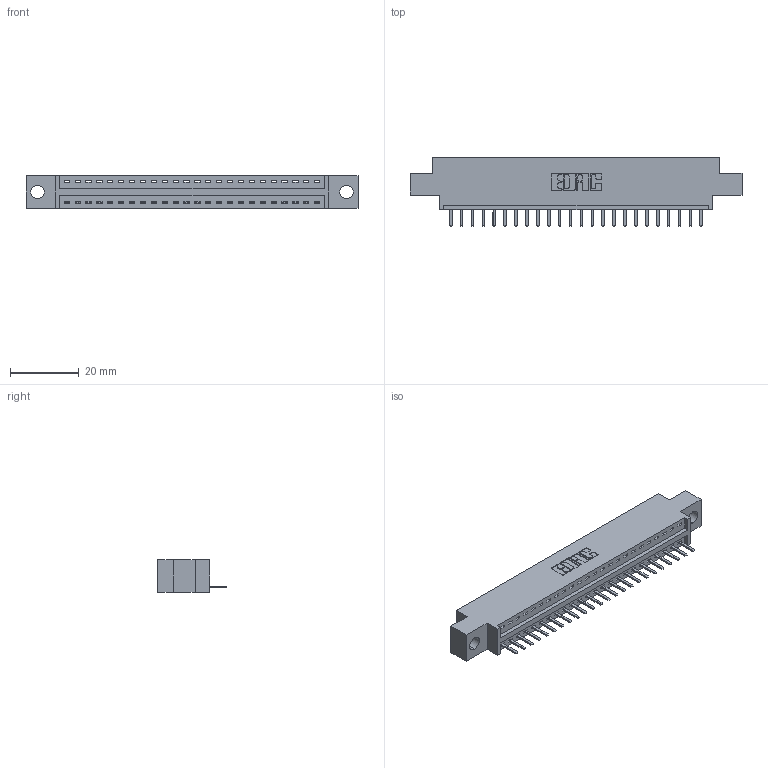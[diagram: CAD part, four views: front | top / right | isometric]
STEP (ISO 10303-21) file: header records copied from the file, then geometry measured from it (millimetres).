
FILE_DESCRIPTION (( 'STEP AP203' ), '1' );
FILE_NAME ('346-024-520-604.STEP', '2022-05-05T22:23:46', ( '' ), ( '' ), 'SwSTEP 2.0', 'SolidWorks 2020', '' );
FILE_SCHEMA (( 'CONFIG_CONTROL_DESIGN' ));
Length unit declared in the file: inch
Products named in the file (3): 346 Part_0.170 Offset - 0.156 Dia-TH; 346-024-520-604; 345-292-001_345-293-120
Assembly tree (25 placements, depth 2):
  346-024-520-604
    346 Part_0.170 Offset - 0.156 Dia-TH
    345-292-001_345-293-120  x24
Bounding box: 96.77 x 20.02 x 9.4 mm (x, y, z)
Volume: 8809.8 mm3; surface area: 10584 mm2
Topology: 25 solids, 25 shells, 1628 faces, 4793 edges, 3130 vertices
Faces by surface type: plane 1102, cylinder 526
Entity records: 17983 total; most frequent: CARTESIAN_POINT 3110, ORIENTED_EDGE 3054, DIRECTION 2751, EDGE_CURVE 1527, LINE 1295, VECTOR 1295, VERTEX_POINT 1014, AXIS2_PLACEMENT_3D 728
